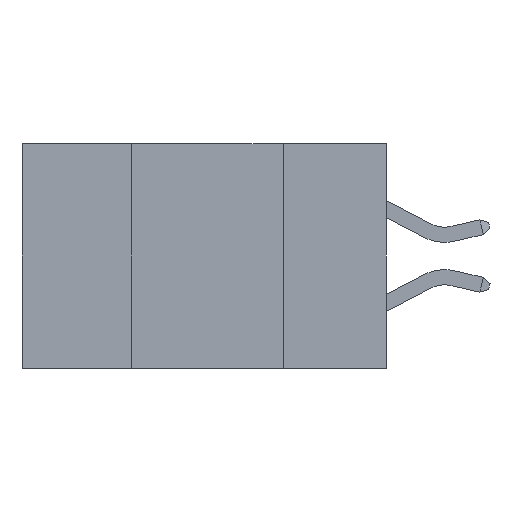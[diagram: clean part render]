
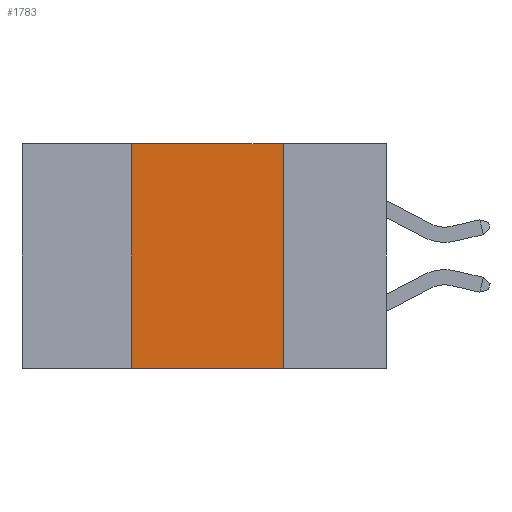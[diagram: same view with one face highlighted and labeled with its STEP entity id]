
A CAD part, left-side view. The second image highlights one B-rep face of the part: STEP entity #1783.
In plain terms, the highlighted planar face has unit normal (-1, 0, 0).
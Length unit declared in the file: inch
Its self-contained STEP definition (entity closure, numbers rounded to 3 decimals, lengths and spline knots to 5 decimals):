
#817 = ORIENTED_EDGE ( 'NONE', *, *, #2743, .F. ) ;
#923 = CARTESIAN_POINT ( 'NONE',  ( 0., 0.42, -0.37 ) ) ;
#1004 = EDGE_LOOP ( 'NONE', ( #1905, #3316, #817, #9000 ) ) ;
#1076 = LINE ( 'NONE', #4309, #9472 ) ;
#1783 = ADVANCED_FACE ( 'NONE', ( #11382 ), #9240, .F. ) ;
#1892 = DIRECTION ( 'NONE',  ( 0., 0., 1. ) ) ;
#1905 = ORIENTED_EDGE ( 'NONE', *, *, #14279, .F. ) ;
#1989 = LINE ( 'NONE', #8330, #10706 ) ;
#2176 = CARTESIAN_POINT ( 'NONE',  ( 0., 0.42, -0.37 ) ) ;
#2743 = EDGE_CURVE ( 'NONE', #7241, #5555, #10300, .T. ) ;
#3196 = VECTOR ( 'NONE', #6700, 39.37008 ) ;
#3316 = ORIENTED_EDGE ( 'NONE', *, *, #5005, .F. ) ;
#3939 = CARTESIAN_POINT ( 'NONE',  ( 0., 0.17, 0. ) ) ;
#4309 = CARTESIAN_POINT ( 'NONE',  ( 0., 0.6, -0.37 ) ) ;
#4431 = CARTESIAN_POINT ( 'NONE',  ( 0., 0.6, 0. ) ) ;
#5005 = EDGE_CURVE ( 'NONE', #5555, #8921, #6201, .T. ) ;
#5555 = VERTEX_POINT ( 'NONE', #11072 ) ;
#6048 = DIRECTION ( 'NONE',  ( 0., 0., -1. ) ) ;
#6201 = LINE ( 'NONE', #4431, #3196 ) ;
#6700 = DIRECTION ( 'NONE',  ( 0., -1., 0. ) ) ;
#7241 = VERTEX_POINT ( 'NONE', #923 ) ;
#7256 = VECTOR ( 'NONE', #1892, 39.37008 ) ;
#7894 = AXIS2_PLACEMENT_3D ( 'NONE', #14198, #8048, #6048 ) ;
#7956 = CARTESIAN_POINT ( 'NONE',  ( 0., 0.17, -0.37 ) ) ;
#8048 = DIRECTION ( 'NONE',  ( 1., 0., 0. ) ) ;
#8330 = CARTESIAN_POINT ( 'NONE',  ( 0., 0.17, -0.37 ) ) ;
#8921 = VERTEX_POINT ( 'NONE', #3939 ) ;
#9000 = ORIENTED_EDGE ( 'NONE', *, *, #14595, .T. ) ;
#9240 = PLANE ( 'NONE',  #7894 ) ;
#9472 = VECTOR ( 'NONE', #11106, 39.37008 ) ;
#9492 = DIRECTION ( 'NONE',  ( 0., 0., -1. ) ) ;
#10300 = LINE ( 'NONE', #2176, #7256 ) ;
#10706 = VECTOR ( 'NONE', #9492, 39.37008 ) ;
#11072 = CARTESIAN_POINT ( 'NONE',  ( 0., 0.42, 0. ) ) ;
#11106 = DIRECTION ( 'NONE',  ( 0., -1., 0. ) ) ;
#11163 = VERTEX_POINT ( 'NONE', #7956 ) ;
#11382 = FACE_OUTER_BOUND ( 'NONE', #1004, .T. ) ;
#14198 = CARTESIAN_POINT ( 'NONE',  ( 0., 0.6, 0. ) ) ;
#14279 = EDGE_CURVE ( 'NONE', #8921, #11163, #1989, .T. ) ;
#14595 = EDGE_CURVE ( 'NONE', #7241, #11163, #1076, .T. ) ;
